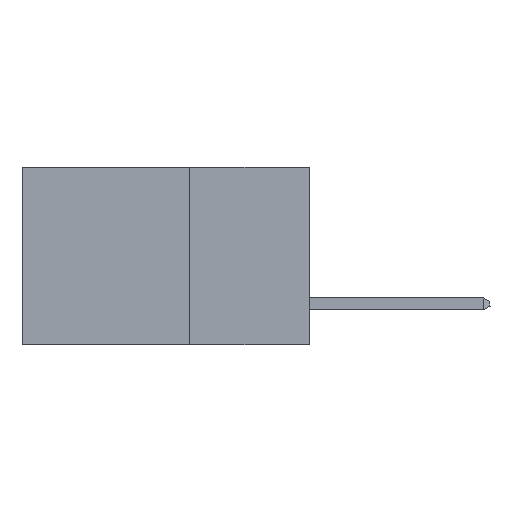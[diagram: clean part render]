
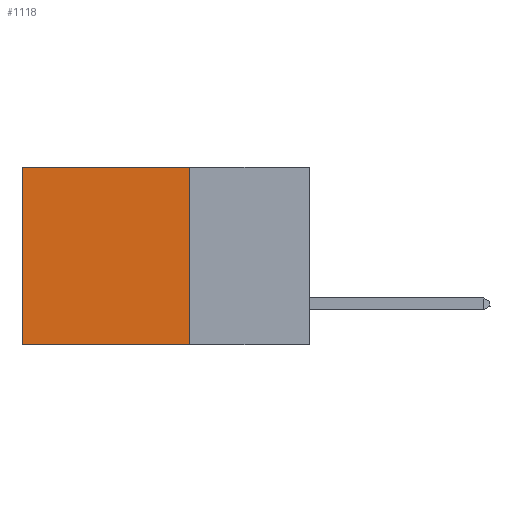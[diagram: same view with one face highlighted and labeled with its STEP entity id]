
A CAD part, left-side view. The second image highlights one B-rep face of the part: STEP entity #1118.
In plain terms, the highlighted planar face has unit normal (-1, 0, 0).
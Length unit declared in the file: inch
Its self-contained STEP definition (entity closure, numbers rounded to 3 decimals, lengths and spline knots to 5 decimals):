
#102 = CARTESIAN_POINT ( 'NONE',  ( 0.2875, 0.25, 0. ) ) ;
#1118 = ADVANCED_FACE ( 'NONE', ( #1526 ), #9726, .F. ) ;
#1526 = FACE_OUTER_BOUND ( 'NONE', #28037, .T. ) ;
#2994 = CARTESIAN_POINT ( 'NONE',  ( 0.2875, 0.25, 0. ) ) ;
#3093 = LINE ( 'NONE', #25457, #8906 ) ;
#3266 = DIRECTION ( 'NONE',  ( 0., 0., -1. ) ) ;
#3437 = CARTESIAN_POINT ( 'NONE',  ( 0.2875, 0.6, 0. ) ) ;
#6029 = CARTESIAN_POINT ( 'NONE',  ( 0.2875, 0.25, -0.37 ) ) ;
#7139 = DIRECTION ( 'NONE',  ( 0., 0., -1. ) ) ;
#8905 = DIRECTION ( 'NONE',  ( 0., 1., 0. ) ) ;
#8906 = VECTOR ( 'NONE', #3266, 39.37008 ) ;
#9433 = CARTESIAN_POINT ( 'NONE',  ( 0.2875, 0.6, -0.37 ) ) ;
#9726 = PLANE ( 'NONE',  #13072 ) ;
#10108 = VERTEX_POINT ( 'NONE', #9433 ) ;
#11194 = VERTEX_POINT ( 'NONE', #26112 ) ;
#13065 = VECTOR ( 'NONE', #24970, 39.37008 ) ;
#13072 = AXIS2_PLACEMENT_3D ( 'NONE', #102, #26732, #7139 ) ;
#15623 = EDGE_CURVE ( 'NONE', #11194, #10108, #22766, .T. ) ;
#16125 = CARTESIAN_POINT ( 'NONE',  ( 0.2875, 0.25, 0. ) ) ;
#16193 = VECTOR ( 'NONE', #8905, 39.37008 ) ;
#16396 = DIRECTION ( 'NONE',  ( 0., 1., 0. ) ) ;
#17253 = ORIENTED_EDGE ( 'NONE', *, *, #17507, .F. ) ;
#17507 = EDGE_CURVE ( 'NONE', #22310, #11194, #27189, .T. ) ;
#19630 = CARTESIAN_POINT ( 'NONE',  ( 0.2875, 0.25, 0. ) ) ;
#20010 = ORIENTED_EDGE ( 'NONE', *, *, #15623, .F. ) ;
#20082 = ORIENTED_EDGE ( 'NONE', *, *, #28561, .T. ) ;
#21971 = ORIENTED_EDGE ( 'NONE', *, *, #27758, .T. ) ;
#22310 = VERTEX_POINT ( 'NONE', #19630 ) ;
#22766 = LINE ( 'NONE', #6029, #31109 ) ;
#24970 = DIRECTION ( 'NONE',  ( 0., 0., -1. ) ) ;
#25457 = CARTESIAN_POINT ( 'NONE',  ( 0.2875, 0.6, 0. ) ) ;
#26112 = CARTESIAN_POINT ( 'NONE',  ( 0.2875, 0.25, -0.37 ) ) ;
#26732 = DIRECTION ( 'NONE',  ( 1., 0., 0. ) ) ;
#27106 = VERTEX_POINT ( 'NONE', #3437 ) ;
#27189 = LINE ( 'NONE', #2994, #13065 ) ;
#27758 = EDGE_CURVE ( 'NONE', #22310, #27106, #30620, .T. ) ;
#28037 = EDGE_LOOP ( 'NONE', ( #20082, #20010, #17253, #21971 ) ) ;
#28561 = EDGE_CURVE ( 'NONE', #27106, #10108, #3093, .T. ) ;
#30620 = LINE ( 'NONE', #16125, #16193 ) ;
#31109 = VECTOR ( 'NONE', #16396, 39.37008 ) ;
